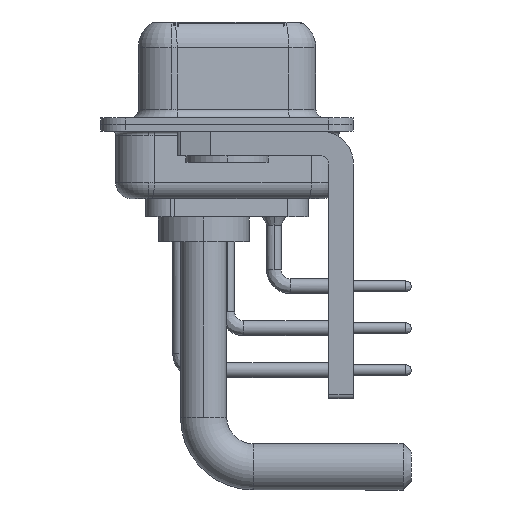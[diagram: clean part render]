
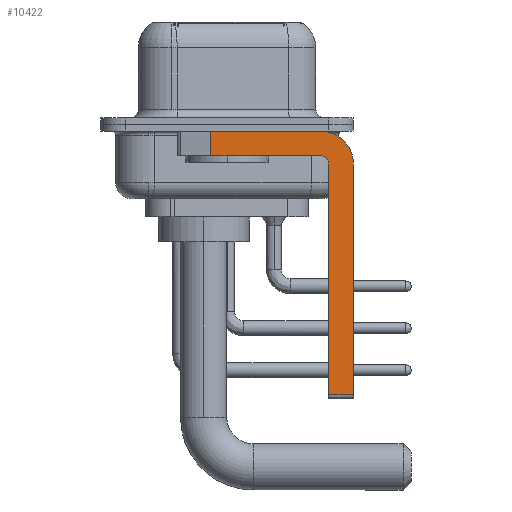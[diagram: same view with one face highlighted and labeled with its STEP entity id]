
A CAD part, left-side view. The second image highlights one B-rep face of the part: STEP entity #10422.
In plain terms, the highlighted planar face has unit normal (-1, 0, 0).
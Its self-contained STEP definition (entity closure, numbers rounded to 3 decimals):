
#852 = CARTESIAN_POINT ( 'NONE',  ( -2.9, -5.65, -0.4 ) ) ;
#1887 = CARTESIAN_POINT ( 'NONE',  ( -2.9, -5.65, -2.4 ) ) ;
#1918 = ORIENTED_EDGE ( 'NONE', *, *, #3039, .F. ) ;
#3039 = EDGE_CURVE ( 'NONE', #33161, #24623, #16592, .T. ) ;
#3378 = CARTESIAN_POINT ( 'NONE',  ( -2.9, -5.65, -1.9 ) ) ;
#3396 = CARTESIAN_POINT ( 'NONE',  ( -2.9, 0.978, -0.4 ) ) ;
#4370 = FACE_OUTER_BOUND ( 'NONE', #27524, .T. ) ;
#4656 = CIRCLE ( 'NONE', #19829, 2. ) ;
#4739 = ORIENTED_EDGE ( 'NONE', *, *, #34349, .F. ) ;
#5034 = DIRECTION ( 'NONE',  ( 0., 0., 1. ) ) ;
#5779 = DIRECTION ( 'NONE',  ( 0., 0., 1. ) ) ;
#6199 = LINE ( 'NONE', #9182, #31202 ) ;
#7046 = VERTEX_POINT ( 'NONE', #852 ) ;
#7166 = DIRECTION ( 'NONE',  ( 0., 0., -1. ) ) ;
#7313 = CARTESIAN_POINT ( 'NONE',  ( -2.9, 0.978, -1.9 ) ) ;
#7736 = CARTESIAN_POINT ( 'NONE',  ( -2.9, -6.15, -2.4 ) ) ;
#8155 = EDGE_CURVE ( 'NONE', #18376, #11225, #22132, .T. ) ;
#8657 = LINE ( 'NONE', #3378, #13286 ) ;
#8771 = CARTESIAN_POINT ( 'NONE',  ( -2.9, -6.15, -16.6 ) ) ;
#9051 = CARTESIAN_POINT ( 'NONE',  ( -2.9, -7.65, -16.35 ) ) ;
#9182 = CARTESIAN_POINT ( 'NONE',  ( -2.9, 3., -0.4 ) ) ;
#10043 = EDGE_CURVE ( 'NONE', #19182, #17040, #32842, .T. ) ;
#10174 = CARTESIAN_POINT ( 'NONE',  ( -2.9, -5.65, -2.4 ) ) ;
#10323 = DIRECTION ( 'NONE',  ( -1., 0., 0. ) ) ;
#10422 = ADVANCED_FACE ( 'NONE', ( #4370 ), #31274, .F. ) ;
#10459 = ORIENTED_EDGE ( 'NONE', *, *, #10043, .T. ) ;
#10944 = CARTESIAN_POINT ( 'NONE',  ( -2.9, -5.65, -1.9 ) ) ;
#11149 = CARTESIAN_POINT ( 'NONE',  ( -2.9, -7.65, -2.4 ) ) ;
#11225 = VERTEX_POINT ( 'NONE', #7736 ) ;
#12179 = DIRECTION ( 'NONE',  ( 0., -1., 0. ) ) ;
#12316 = CARTESIAN_POINT ( 'NONE',  ( -2.9, -7.65, -2.4 ) ) ;
#13286 = VECTOR ( 'NONE', #30117, 1000. ) ;
#13863 = DIRECTION ( 'NONE',  ( 0., 0., -1. ) ) ;
#16221 = CARTESIAN_POINT ( 'NONE',  ( -2.9, -5.65, -2.4 ) ) ;
#16592 = LINE ( 'NONE', #11149, #30765 ) ;
#17040 = VERTEX_POINT ( 'NONE', #7313 ) ;
#17130 = CARTESIAN_POINT ( 'NONE',  ( -2.9, -5.65, -16.35 ) ) ;
#17679 = AXIS2_PLACEMENT_3D ( 'NONE', #1887, #10323, #5034 ) ;
#18352 = DIRECTION ( 'NONE',  ( 1., 0., 0. ) ) ;
#18376 = VERTEX_POINT ( 'NONE', #29480 ) ;
#19143 = ORIENTED_EDGE ( 'NONE', *, *, #32242, .F. ) ;
#19182 = VERTEX_POINT ( 'NONE', #3396 ) ;
#19645 = ORIENTED_EDGE ( 'NONE', *, *, #20503, .F. ) ;
#19777 = EDGE_CURVE ( 'NONE', #11225, #34303, #32801, .T. ) ;
#19829 = AXIS2_PLACEMENT_3D ( 'NONE', #16221, #18352, #29102 ) ;
#20400 = DIRECTION ( 'NONE',  ( 1., 0., 0. ) ) ;
#20503 = EDGE_CURVE ( 'NONE', #19182, #7046, #6199, .T. ) ;
#21076 = ORIENTED_EDGE ( 'NONE', *, *, #8155, .F. ) ;
#22048 = DIRECTION ( 'NONE',  ( 0., 0., -1. ) ) ;
#22132 = LINE ( 'NONE', #8771, #27644 ) ;
#23321 = VECTOR ( 'NONE', #13863, 1000. ) ;
#24623 = VERTEX_POINT ( 'NONE', #9051 ) ;
#24990 = ORIENTED_EDGE ( 'NONE', *, *, #29618, .T. ) ;
#27524 = EDGE_LOOP ( 'NONE', ( #19645, #10459, #4739, #32650, #21076, #24990, #1918, #19143 ) ) ;
#27644 = VECTOR ( 'NONE', #5779, 1000. ) ;
#29102 = DIRECTION ( 'NONE',  ( 0., 0., -1. ) ) ;
#29480 = CARTESIAN_POINT ( 'NONE',  ( -2.9, -6.15, -16.35 ) ) ;
#29618 = EDGE_CURVE ( 'NONE', #18376, #24623, #32447, .T. ) ;
#29894 = CARTESIAN_POINT ( 'NONE',  ( -2.9, 0.978, -1.9 ) ) ;
#30117 = DIRECTION ( 'NONE',  ( 0., 1., 0. ) ) ;
#30765 = VECTOR ( 'NONE', #22048, 1000. ) ;
#30942 = VECTOR ( 'NONE', #12179, 1000. ) ;
#31202 = VECTOR ( 'NONE', #33098, 1000. ) ;
#31274 = PLANE ( 'NONE',  #34622 ) ;
#32242 = EDGE_CURVE ( 'NONE', #7046, #33161, #4656, .T. ) ;
#32447 = LINE ( 'NONE', #17130, #30942 ) ;
#32650 = ORIENTED_EDGE ( 'NONE', *, *, #19777, .F. ) ;
#32801 = CIRCLE ( 'NONE', #17679, 0.5 ) ;
#32842 = LINE ( 'NONE', #29894, #23321 ) ;
#33098 = DIRECTION ( 'NONE',  ( 0., -1., 0. ) ) ;
#33161 = VERTEX_POINT ( 'NONE', #12316 ) ;
#34303 = VERTEX_POINT ( 'NONE', #10944 ) ;
#34349 = EDGE_CURVE ( 'NONE', #34303, #17040, #8657, .T. ) ;
#34622 = AXIS2_PLACEMENT_3D ( 'NONE', #10174, #20400, #7166 ) ;
